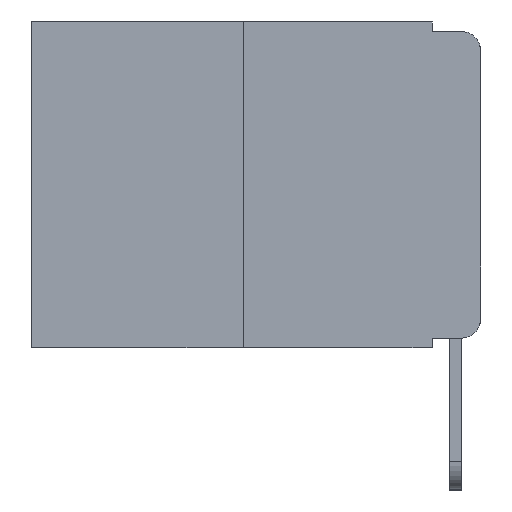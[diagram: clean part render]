
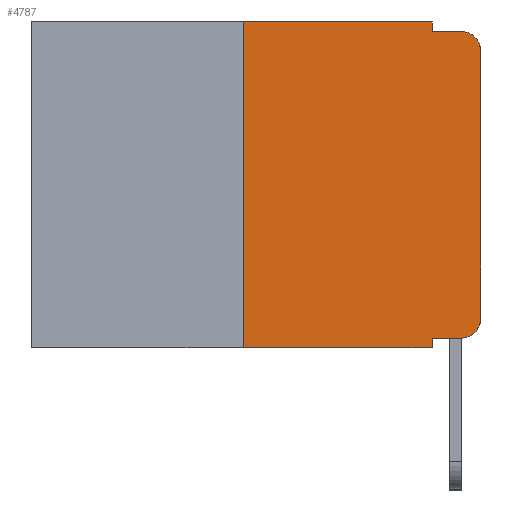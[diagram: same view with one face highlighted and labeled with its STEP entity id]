
A CAD part, left-side view. The second image highlights one B-rep face of the part: STEP entity #4787.
In plain terms, the highlighted planar face has unit normal (-1, 0, 0).
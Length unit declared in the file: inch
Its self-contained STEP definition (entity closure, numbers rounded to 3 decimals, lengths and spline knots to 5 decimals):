
#275 = VECTOR ( 'NONE', #8367, 39.37008 ) ;
#319 = CARTESIAN_POINT ( 'NONE',  ( 0., 0.02, -0.01 ) ) ;
#376 = LINE ( 'NONE', #7716, #2950 ) ;
#488 = CARTESIAN_POINT ( 'NONE',  ( 0., 0.02, -0.313 ) ) ;
#494 = ORIENTED_EDGE ( 'NONE', *, *, #6586, .T. ) ;
#593 = EDGE_CURVE ( 'NONE', #3595, #7363, #1458, .T. ) ;
#684 = CARTESIAN_POINT ( 'NONE',  ( 0., 0.051, -0.343 ) ) ;
#1458 = LINE ( 'NONE', #12481, #7308 ) ;
#1519 = EDGE_CURVE ( 'NONE', #6342, #7524, #12752, .T. ) ;
#1861 = EDGE_CURVE ( 'NONE', #4307, #7696, #10875, .T. ) ;
#1925 = VERTEX_POINT ( 'NONE', #4264 ) ;
#2204 = VERTEX_POINT ( 'NONE', #684 ) ;
#2234 = CARTESIAN_POINT ( 'NONE',  ( 0., 0.02, -0.03 ) ) ;
#2470 = EDGE_CURVE ( 'NONE', #7363, #3771, #6760, .T. ) ;
#2514 = EDGE_CURVE ( 'NONE', #3595, #2204, #6079, .T. ) ;
#2656 = DIRECTION ( 'NONE',  ( 0., 0., -1. ) ) ;
#2693 = DIRECTION ( 'NONE',  ( 0., -1., 0. ) ) ;
#2950 = VECTOR ( 'NONE', #13770, 39.37008 ) ;
#3134 = AXIS2_PLACEMENT_3D ( 'NONE', #14023, #4794, #9157 ) ;
#3139 = VECTOR ( 'NONE', #2693, 39.37008 ) ;
#3209 = DIRECTION ( 'NONE',  ( 0., 0., 1. ) ) ;
#3344 = DIRECTION ( 'NONE',  ( 0., 0., -1. ) ) ;
#3486 = VECTOR ( 'NONE', #7532, 39.37008 ) ;
#3547 = PLANE ( 'NONE',  #3134 ) ;
#3595 = VERTEX_POINT ( 'NONE', #13512 ) ;
#3602 = AXIS2_PLACEMENT_3D ( 'NONE', #488, #11694, #2656 ) ;
#3771 = VERTEX_POINT ( 'NONE', #3789 ) ;
#3789 = CARTESIAN_POINT ( 'NONE',  ( 0., 0.051, 0. ) ) ;
#3999 = VECTOR ( 'NONE', #11808, 39.37008 ) ;
#4172 = ORIENTED_EDGE ( 'NONE', *, *, #1861, .T. ) ;
#4264 = CARTESIAN_POINT ( 'NONE',  ( 0., 0., -0.03 ) ) ;
#4307 = VERTEX_POINT ( 'NONE', #13382 ) ;
#4563 = EDGE_CURVE ( 'NONE', #4307, #2204, #6821, .T. ) ;
#4787 = ADVANCED_FACE ( 'NONE', ( #5957 ), #3547, .F. ) ;
#4794 = DIRECTION ( 'NONE',  ( 1., 0., 0. ) ) ;
#5080 = DIRECTION ( 'NONE',  ( 0., 0., -1. ) ) ;
#5088 = CARTESIAN_POINT ( 'NONE',  ( 0., 0., -0.313 ) ) ;
#5109 = EDGE_CURVE ( 'NONE', #7696, #9065, #7306, .T. ) ;
#5957 = FACE_OUTER_BOUND ( 'NONE', #9661, .T. ) ;
#6079 = LINE ( 'NONE', #11060, #3139 ) ;
#6342 = VERTEX_POINT ( 'NONE', #13140 ) ;
#6586 = EDGE_CURVE ( 'NONE', #9065, #1925, #376, .T. ) ;
#6653 = ORIENTED_EDGE ( 'NONE', *, *, #13840, .F. ) ;
#6760 = LINE ( 'NONE', #8747, #3486 ) ;
#6821 = LINE ( 'NONE', #9807, #275 ) ;
#6890 = ORIENTED_EDGE ( 'NONE', *, *, #5109, .T. ) ;
#7166 = ORIENTED_EDGE ( 'NONE', *, *, #2514, .T. ) ;
#7306 = CIRCLE ( 'NONE', #3602, 0.02 ) ;
#7308 = VECTOR ( 'NONE', #3209, 39.37008 ) ;
#7363 = VERTEX_POINT ( 'NONE', #9767 ) ;
#7524 = VERTEX_POINT ( 'NONE', #319 ) ;
#7532 = DIRECTION ( 'NONE',  ( 0., -1., 0. ) ) ;
#7684 = LINE ( 'NONE', #11654, #10955 ) ;
#7696 = VERTEX_POINT ( 'NONE', #12645 ) ;
#7709 = CARTESIAN_POINT ( 'NONE',  ( 0., 0.051, -0.01 ) ) ;
#7716 = CARTESIAN_POINT ( 'NONE',  ( 0., 0., 0. ) ) ;
#7955 = VECTOR ( 'NONE', #8801, 39.37008 ) ;
#8188 = ORIENTED_EDGE ( 'NONE', *, *, #2470, .F. ) ;
#8367 = DIRECTION ( 'NONE',  ( 0., 0., -1. ) ) ;
#8747 = CARTESIAN_POINT ( 'NONE',  ( 0., 0.473, 0. ) ) ;
#8801 = DIRECTION ( 'NONE',  ( 0., -1., 0. ) ) ;
#9065 = VERTEX_POINT ( 'NONE', #5088 ) ;
#9157 = DIRECTION ( 'NONE',  ( 0., 0., -1. ) ) ;
#9661 = EDGE_LOOP ( 'NONE', ( #494, #13703, #14220, #6653, #8188, #11336, #7166, #14210, #4172, #6890 ) ) ;
#9767 = CARTESIAN_POINT ( 'NONE',  ( 0., 0.25, 0. ) ) ;
#9807 = CARTESIAN_POINT ( 'NONE',  ( 0., 0.051, 0. ) ) ;
#9922 = DIRECTION ( 'NONE',  ( -1., 0., 0. ) ) ;
#10875 = LINE ( 'NONE', #12530, #7955 ) ;
#10955 = VECTOR ( 'NONE', #5080, 39.37008 ) ;
#11060 = CARTESIAN_POINT ( 'NONE',  ( 0., 0.473, -0.343 ) ) ;
#11107 = EDGE_CURVE ( 'NONE', #1925, #7524, #13093, .T. ) ;
#11336 = ORIENTED_EDGE ( 'NONE', *, *, #593, .F. ) ;
#11576 = AXIS2_PLACEMENT_3D ( 'NONE', #2234, #9922, #3344 ) ;
#11654 = CARTESIAN_POINT ( 'NONE',  ( 0., 0.051, 0. ) ) ;
#11694 = DIRECTION ( 'NONE',  ( -1., 0., 0. ) ) ;
#11808 = DIRECTION ( 'NONE',  ( 0., -1., 0. ) ) ;
#12481 = CARTESIAN_POINT ( 'NONE',  ( 0., 0.25, 0. ) ) ;
#12530 = CARTESIAN_POINT ( 'NONE',  ( 0., 0.051, -0.333 ) ) ;
#12645 = CARTESIAN_POINT ( 'NONE',  ( 0., 0.02, -0.333 ) ) ;
#12752 = LINE ( 'NONE', #7709, #3999 ) ;
#13093 = CIRCLE ( 'NONE', #11576, 0.02 ) ;
#13140 = CARTESIAN_POINT ( 'NONE',  ( 0., 0.051, -0.01 ) ) ;
#13382 = CARTESIAN_POINT ( 'NONE',  ( 0., 0.051, -0.333 ) ) ;
#13512 = CARTESIAN_POINT ( 'NONE',  ( 0., 0.25, -0.343 ) ) ;
#13703 = ORIENTED_EDGE ( 'NONE', *, *, #11107, .T. ) ;
#13770 = DIRECTION ( 'NONE',  ( 0., 0., 1. ) ) ;
#13840 = EDGE_CURVE ( 'NONE', #3771, #6342, #7684, .T. ) ;
#14023 = CARTESIAN_POINT ( 'NONE',  ( 0., 0.473, 0. ) ) ;
#14210 = ORIENTED_EDGE ( 'NONE', *, *, #4563, .F. ) ;
#14220 = ORIENTED_EDGE ( 'NONE', *, *, #1519, .F. ) ;
